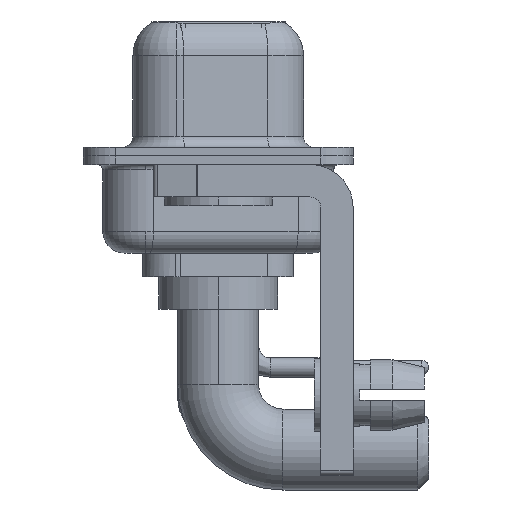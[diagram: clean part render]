
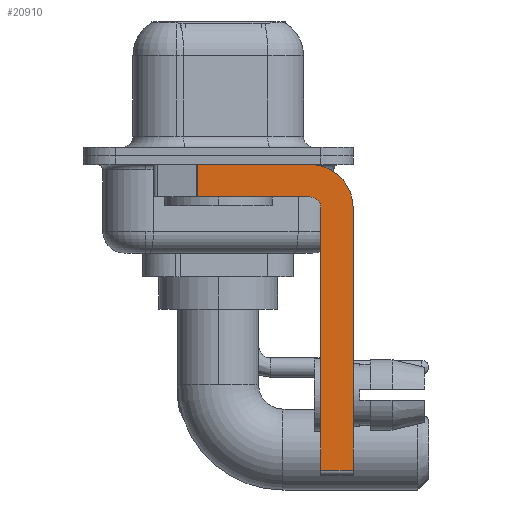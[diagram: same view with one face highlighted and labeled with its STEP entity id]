
A CAD part, left-side view. The second image highlights one B-rep face of the part: STEP entity #20910.
In plain terms, the highlighted planar face has unit normal (-1, 0, 0).
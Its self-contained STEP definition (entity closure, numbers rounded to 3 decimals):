
#36 = CARTESIAN_POINT ( 'NONE',  ( -2.9, 0.978, -1.9 ) ) ;
#175 = DIRECTION ( 'NONE',  ( 0., 0., 1. ) ) ;
#357 = DIRECTION ( 'NONE',  ( 0., 1., 0. ) ) ;
#769 = LINE ( 'NONE', #11298, #8383 ) ;
#835 = CARTESIAN_POINT ( 'NONE',  ( -2.9, -4.25, -2.4 ) ) ;
#905 = EDGE_LOOP ( 'NONE', ( #16570, #12817, #8245, #8284, #21582, #5658, #2733, #3995 ) ) ;
#1264 = DIRECTION ( 'NONE',  ( 0., 0., -1. ) ) ;
#1296 = VERTEX_POINT ( 'NONE', #2929 ) ;
#1700 = LINE ( 'NONE', #17474, #6916 ) ;
#2733 = ORIENTED_EDGE ( 'NONE', *, *, #16350, .F. ) ;
#2819 = EDGE_CURVE ( 'NONE', #1296, #17443, #10894, .T. ) ;
#2929 = CARTESIAN_POINT ( 'NONE',  ( -2.9, -4.25, -0.4 ) ) ;
#3343 = VECTOR ( 'NONE', #357, 1000. ) ;
#3732 = EDGE_CURVE ( 'NONE', #20698, #16013, #17525, .T. ) ;
#3995 = ORIENTED_EDGE ( 'NONE', *, *, #2819, .F. ) ;
#4225 = VECTOR ( 'NONE', #175, 1000. ) ;
#4492 = AXIS2_PLACEMENT_3D ( 'NONE', #835, #17149, #1264 ) ;
#4563 = DIRECTION ( 'NONE',  ( 0., -1., 0. ) ) ;
#4801 = CARTESIAN_POINT ( 'NONE',  ( -2.9, -6.25, -2.4 ) ) ;
#5146 = EDGE_CURVE ( 'NONE', #5458, #20698, #10690, .T. ) ;
#5458 = VERTEX_POINT ( 'NONE', #6770 ) ;
#5658 = ORIENTED_EDGE ( 'NONE', *, *, #10744, .T. ) ;
#6055 = LINE ( 'NONE', #21703, #13872 ) ;
#6770 = CARTESIAN_POINT ( 'NONE',  ( -2.9, -4.75, -14.55 ) ) ;
#6794 = DIRECTION ( 'NONE',  ( 0., 0., 1. ) ) ;
#6817 = VERTEX_POINT ( 'NONE', #36 ) ;
#6916 = VECTOR ( 'NONE', #10386, 1000. ) ;
#6923 = CARTESIAN_POINT ( 'NONE',  ( -2.9, -4.25, -2.4 ) ) ;
#8245 = ORIENTED_EDGE ( 'NONE', *, *, #13181, .F. ) ;
#8284 = ORIENTED_EDGE ( 'NONE', *, *, #3732, .F. ) ;
#8315 = CARTESIAN_POINT ( 'NONE',  ( -2.9, 0.978, -1.9 ) ) ;
#8362 = VECTOR ( 'NONE', #13465, 1000. ) ;
#8383 = VECTOR ( 'NONE', #19745, 1000. ) ;
#8389 = CARTESIAN_POINT ( 'NONE',  ( -2.9, -4.25, -2.4 ) ) ;
#9172 = CARTESIAN_POINT ( 'NONE',  ( -2.9, -4.75, -2.4 ) ) ;
#9570 = EDGE_CURVE ( 'NONE', #12356, #6817, #15399, .T. ) ;
#10123 = DIRECTION ( 'NONE',  ( 0., 0., -1. ) ) ;
#10386 = DIRECTION ( 'NONE',  ( 0., 0., -1. ) ) ;
#10596 = AXIS2_PLACEMENT_3D ( 'NONE', #8389, #22449, #6794 ) ;
#10690 = LINE ( 'NONE', #12406, #4225 ) ;
#10744 = EDGE_CURVE ( 'NONE', #5458, #11976, #6055, .T. ) ;
#10894 = CIRCLE ( 'NONE', #11253, 2. ) ;
#11253 = AXIS2_PLACEMENT_3D ( 'NONE', #6923, #17105, #10123 ) ;
#11298 = CARTESIAN_POINT ( 'NONE',  ( -2.9, 3., -0.4 ) ) ;
#11976 = VERTEX_POINT ( 'NONE', #18817 ) ;
#12356 = VERTEX_POINT ( 'NONE', #14554 ) ;
#12406 = CARTESIAN_POINT ( 'NONE',  ( -2.9, -4.75, -14.8 ) ) ;
#12817 = ORIENTED_EDGE ( 'NONE', *, *, #9570, .T. ) ;
#13181 = EDGE_CURVE ( 'NONE', #16013, #6817, #21278, .T. ) ;
#13465 = DIRECTION ( 'NONE',  ( 0., 0., -1. ) ) ;
#13872 = VECTOR ( 'NONE', #4563, 1000. ) ;
#14554 = CARTESIAN_POINT ( 'NONE',  ( -2.9, 0.978, -0.4 ) ) ;
#15399 = LINE ( 'NONE', #8315, #8362 ) ;
#15913 = CARTESIAN_POINT ( 'NONE',  ( -2.9, -4.25, -1.9 ) ) ;
#16013 = VERTEX_POINT ( 'NONE', #18289 ) ;
#16350 = EDGE_CURVE ( 'NONE', #17443, #11976, #1700, .T. ) ;
#16449 = EDGE_CURVE ( 'NONE', #12356, #1296, #769, .T. ) ;
#16570 = ORIENTED_EDGE ( 'NONE', *, *, #16449, .F. ) ;
#17105 = DIRECTION ( 'NONE',  ( 1., 0., 0. ) ) ;
#17149 = DIRECTION ( 'NONE',  ( 1., 0., 0. ) ) ;
#17443 = VERTEX_POINT ( 'NONE', #4801 ) ;
#17474 = CARTESIAN_POINT ( 'NONE',  ( -2.9, -6.25, -2.4 ) ) ;
#17525 = CIRCLE ( 'NONE', #10596, 0.5 ) ;
#18289 = CARTESIAN_POINT ( 'NONE',  ( -2.9, -4.25, -1.9 ) ) ;
#18759 = PLANE ( 'NONE',  #4492 ) ;
#18817 = CARTESIAN_POINT ( 'NONE',  ( -2.9, -6.25, -14.55 ) ) ;
#19745 = DIRECTION ( 'NONE',  ( 0., -1., 0. ) ) ;
#20698 = VERTEX_POINT ( 'NONE', #9172 ) ;
#20910 = ADVANCED_FACE ( 'NONE', ( #22183 ), #18759, .F. ) ;
#21278 = LINE ( 'NONE', #15913, #3343 ) ;
#21582 = ORIENTED_EDGE ( 'NONE', *, *, #5146, .F. ) ;
#21703 = CARTESIAN_POINT ( 'NONE',  ( -2.9, -4.25, -14.55 ) ) ;
#22183 = FACE_OUTER_BOUND ( 'NONE', #905, .T. ) ;
#22449 = DIRECTION ( 'NONE',  ( -1., 0., 0. ) ) ;
